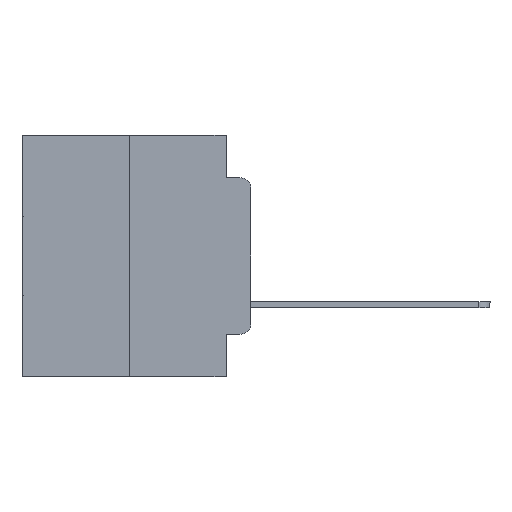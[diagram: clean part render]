
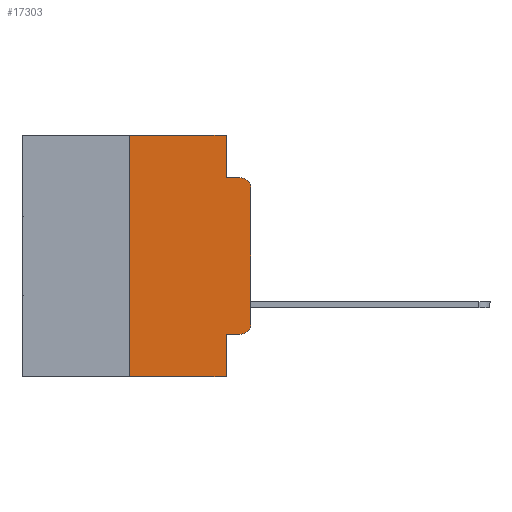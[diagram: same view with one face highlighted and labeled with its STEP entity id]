
A CAD part, left-side view. The second image highlights one B-rep face of the part: STEP entity #17303.
In plain terms, the highlighted planar face has unit normal (-1, 0, 0).
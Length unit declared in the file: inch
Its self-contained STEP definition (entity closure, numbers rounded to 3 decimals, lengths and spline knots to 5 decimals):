
#255 = AXIS2_PLACEMENT_3D ( 'NONE', #23255, #336, #7420 ) ;
#336 = DIRECTION ( 'NONE',  ( -1., 0., 0. ) ) ;
#709 = LINE ( 'NONE', #8097, #9353 ) ;
#1417 = VERTEX_POINT ( 'NONE', #21033 ) ;
#1740 = DIRECTION ( 'NONE',  ( 0., -1., 0. ) ) ;
#2432 = DIRECTION ( 'NONE',  ( 0., 0., 1. ) ) ;
#2725 = EDGE_CURVE ( 'NONE', #11736, #26200, #24666, .T. ) ;
#2775 = CARTESIAN_POINT ( 'NONE',  ( 0., 0.02, -0.1085 ) ) ;
#3317 = DIRECTION ( 'NONE',  ( 1., 0., 0. ) ) ;
#3553 = ORIENTED_EDGE ( 'NONE', *, *, #16002, .T. ) ;
#3615 = VECTOR ( 'NONE', #1740, 39.37008 ) ;
#3985 = CARTESIAN_POINT ( 'NONE',  ( 0., 0.051, -0.0885 ) ) ;
#4698 = CARTESIAN_POINT ( 'NONE',  ( 0., 0.473, -0.5 ) ) ;
#4762 = CARTESIAN_POINT ( 'NONE',  ( 0., 0.473, 0. ) ) ;
#4763 = EDGE_CURVE ( 'NONE', #7838, #26200, #13443, .T. ) ;
#4889 = CARTESIAN_POINT ( 'NONE',  ( 0., 0.051, -0.0885 ) ) ;
#5136 = ORIENTED_EDGE ( 'NONE', *, *, #13015, .F. ) ;
#5138 = AXIS2_PLACEMENT_3D ( 'NONE', #24272, #3317, #12846 ) ;
#5375 = DIRECTION ( 'NONE',  ( 0., 0., -1. ) ) ;
#5893 = VECTOR ( 'NONE', #7002, 39.37008 ) ;
#6243 = VECTOR ( 'NONE', #27731, 39.37008 ) ;
#7002 = DIRECTION ( 'NONE',  ( 0., 0., -1. ) ) ;
#7119 = CARTESIAN_POINT ( 'NONE',  ( 0., 0., 0. ) ) ;
#7137 = ORIENTED_EDGE ( 'NONE', *, *, #10895, .T. ) ;
#7420 = DIRECTION ( 'NONE',  ( 0., 0., -1. ) ) ;
#7527 = CARTESIAN_POINT ( 'NONE',  ( 0., 0.02, -0.0885 ) ) ;
#7708 = PLANE ( 'NONE',  #5138 ) ;
#7838 = VERTEX_POINT ( 'NONE', #26471 ) ;
#7961 = ORIENTED_EDGE ( 'NONE', *, *, #13791, .F. ) ;
#8097 = CARTESIAN_POINT ( 'NONE',  ( 0., 0.25, 0. ) ) ;
#8176 = CARTESIAN_POINT ( 'NONE',  ( 0., 0.051, -0.4115 ) ) ;
#8806 = EDGE_LOOP ( 'NONE', ( #17024, #11661, #22718, #7961, #18102, #22713, #7137, #5136, #28871, #3553 ) ) ;
#8965 = LINE ( 'NONE', #27677, #5893 ) ;
#9353 = VECTOR ( 'NONE', #14301, 39.37008 ) ;
#9612 = LINE ( 'NONE', #14889, #27615 ) ;
#10039 = DIRECTION ( 'NONE',  ( -1., 0., 0. ) ) ;
#10586 = LINE ( 'NONE', #4762, #6243 ) ;
#10895 = EDGE_CURVE ( 'NONE', #1417, #22491, #25399, .T. ) ;
#11661 = ORIENTED_EDGE ( 'NONE', *, *, #4763, .T. ) ;
#11736 = VERTEX_POINT ( 'NONE', #4889 ) ;
#12295 = DIRECTION ( 'NONE',  ( 0., -1., 0. ) ) ;
#12846 = DIRECTION ( 'NONE',  ( 0., 0., -1. ) ) ;
#12871 = CARTESIAN_POINT ( 'NONE',  ( 0., 0.051, 0. ) ) ;
#13015 = EDGE_CURVE ( 'NONE', #14192, #22491, #8965, .T. ) ;
#13443 = CIRCLE ( 'NONE', #21127, 0.02 ) ;
#13791 = EDGE_CURVE ( 'NONE', #21520, #11736, #9612, .T. ) ;
#14112 = CARTESIAN_POINT ( 'NONE',  ( 0., 0., -0.3915 ) ) ;
#14192 = VERTEX_POINT ( 'NONE', #28294 ) ;
#14301 = DIRECTION ( 'NONE',  ( 0., 0., 1. ) ) ;
#14518 = LINE ( 'NONE', #7119, #21504 ) ;
#14889 = CARTESIAN_POINT ( 'NONE',  ( 0., 0.051, 0. ) ) ;
#15105 = EDGE_CURVE ( 'NONE', #1417, #20960, #709, .T. ) ;
#15640 = VERTEX_POINT ( 'NONE', #22083 ) ;
#15699 = VECTOR ( 'NONE', #17370, 39.37008 ) ;
#16002 = EDGE_CURVE ( 'NONE', #15640, #20833, #20501, .T. ) ;
#16196 = EDGE_CURVE ( 'NONE', #14192, #15640, #19631, .T. ) ;
#16968 = DIRECTION ( 'NONE',  ( 0., 0., -1. ) ) ;
#17024 = ORIENTED_EDGE ( 'NONE', *, *, #27488, .T. ) ;
#17303 = ADVANCED_FACE ( 'NONE', ( #23994 ), #7708, .F. ) ;
#17370 = DIRECTION ( 'NONE',  ( 0., -1., 0. ) ) ;
#18102 = ORIENTED_EDGE ( 'NONE', *, *, #21694, .F. ) ;
#19631 = LINE ( 'NONE', #8176, #15699 ) ;
#20501 = CIRCLE ( 'NONE', #255, 0.02 ) ;
#20833 = VERTEX_POINT ( 'NONE', #14112 ) ;
#20960 = VERTEX_POINT ( 'NONE', #21497 ) ;
#21033 = CARTESIAN_POINT ( 'NONE',  ( 0., 0.25, -0.5 ) ) ;
#21127 = AXIS2_PLACEMENT_3D ( 'NONE', #2775, #10039, #16968 ) ;
#21497 = CARTESIAN_POINT ( 'NONE',  ( 0., 0.25, 0. ) ) ;
#21504 = VECTOR ( 'NONE', #2432, 39.37008 ) ;
#21520 = VERTEX_POINT ( 'NONE', #12871 ) ;
#21694 = EDGE_CURVE ( 'NONE', #20960, #21520, #10586, .T. ) ;
#22083 = CARTESIAN_POINT ( 'NONE',  ( 0., 0.02, -0.4115 ) ) ;
#22491 = VERTEX_POINT ( 'NONE', #27503 ) ;
#22713 = ORIENTED_EDGE ( 'NONE', *, *, #15105, .F. ) ;
#22718 = ORIENTED_EDGE ( 'NONE', *, *, #2725, .F. ) ;
#23255 = CARTESIAN_POINT ( 'NONE',  ( 0., 0.02, -0.3915 ) ) ;
#23994 = FACE_OUTER_BOUND ( 'NONE', #8806, .T. ) ;
#24272 = CARTESIAN_POINT ( 'NONE',  ( 0., 0.473, 0. ) ) ;
#24666 = LINE ( 'NONE', #3985, #3615 ) ;
#24842 = VECTOR ( 'NONE', #12295, 39.37008 ) ;
#25399 = LINE ( 'NONE', #4698, #24842 ) ;
#26200 = VERTEX_POINT ( 'NONE', #7527 ) ;
#26471 = CARTESIAN_POINT ( 'NONE',  ( 0., 0., -0.1085 ) ) ;
#27488 = EDGE_CURVE ( 'NONE', #20833, #7838, #14518, .T. ) ;
#27503 = CARTESIAN_POINT ( 'NONE',  ( 0., 0.051, -0.5 ) ) ;
#27615 = VECTOR ( 'NONE', #5375, 39.37008 ) ;
#27677 = CARTESIAN_POINT ( 'NONE',  ( 0., 0.051, 0. ) ) ;
#27731 = DIRECTION ( 'NONE',  ( 0., -1., 0. ) ) ;
#28294 = CARTESIAN_POINT ( 'NONE',  ( 0., 0.051, -0.4115 ) ) ;
#28871 = ORIENTED_EDGE ( 'NONE', *, *, #16196, .T. ) ;
